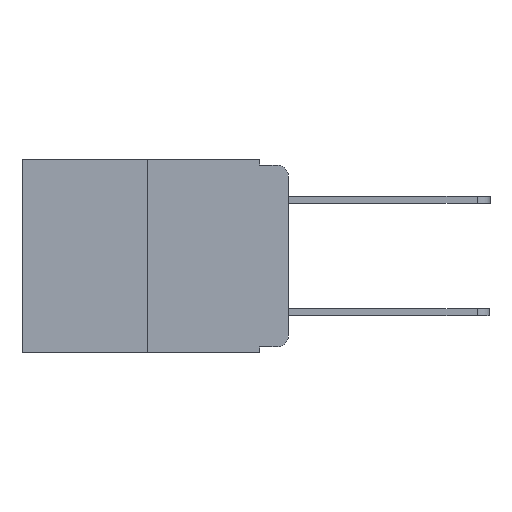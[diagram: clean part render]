
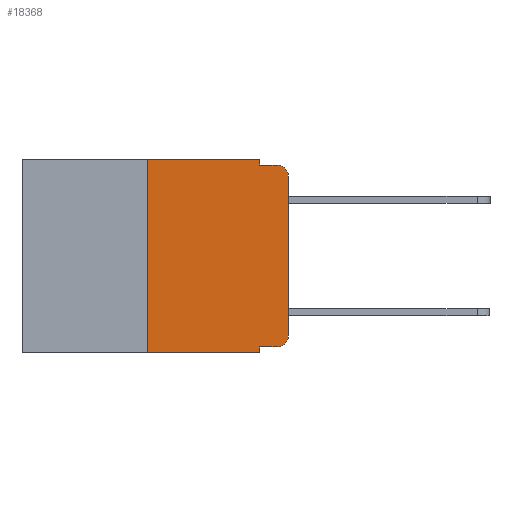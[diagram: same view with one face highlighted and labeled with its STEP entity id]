
A CAD part, left-side view. The second image highlights one B-rep face of the part: STEP entity #18368.
In plain terms, the highlighted planar face has unit normal (-1, 0, 0).
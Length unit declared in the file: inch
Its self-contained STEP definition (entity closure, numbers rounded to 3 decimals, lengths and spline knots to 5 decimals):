
#174 = LINE ( 'NONE', #11953, #8660 ) ;
#197 = DIRECTION ( 'NONE',  ( 0., -1., 0. ) ) ;
#627 = CIRCLE ( 'NONE', #7458, 0.02 ) ;
#633 = FACE_OUTER_BOUND ( 'NONE', #10012, .T. ) ;
#729 = EDGE_CURVE ( 'NONE', #17519, #19519, #13135, .T. ) ;
#1101 = AXIS2_PLACEMENT_3D ( 'NONE', #19298, #20832, #11351 ) ;
#1131 = VECTOR ( 'NONE', #9187, 39.37008 ) ;
#1470 = DIRECTION ( 'NONE',  ( 0., 0., 1. ) ) ;
#1717 = CARTESIAN_POINT ( 'NONE',  ( 0., 0.25, -0.343 ) ) ;
#2043 = ORIENTED_EDGE ( 'NONE', *, *, #7454, .F. ) ;
#2883 = LINE ( 'NONE', #11613, #15964 ) ;
#3343 = CARTESIAN_POINT ( 'NONE',  ( 0., 0.02, -0.03 ) ) ;
#3801 = EDGE_CURVE ( 'NONE', #7958, #6094, #5307, .T. ) ;
#4174 = EDGE_CURVE ( 'NONE', #19519, #8230, #627, .T. ) ;
#4401 = ORIENTED_EDGE ( 'NONE', *, *, #20935, .T. ) ;
#4832 = DIRECTION ( 'NONE',  ( 0., 0., 1. ) ) ;
#4846 = DIRECTION ( 'NONE',  ( -1., 0., 0. ) ) ;
#5013 = DIRECTION ( 'NONE',  ( 0., 0., -1. ) ) ;
#5307 = LINE ( 'NONE', #10705, #13522 ) ;
#5488 = VECTOR ( 'NONE', #1470, 39.37008 ) ;
#5568 = CARTESIAN_POINT ( 'NONE',  ( 0., 0., 0. ) ) ;
#5760 = DIRECTION ( 'NONE',  ( 0., -1., 0. ) ) ;
#5832 = CARTESIAN_POINT ( 'NONE',  ( 0., 0., -0.03 ) ) ;
#6094 = VERTEX_POINT ( 'NONE', #17076 ) ;
#6230 = EDGE_CURVE ( 'NONE', #17071, #16014, #14375, .T. ) ;
#7445 = ORIENTED_EDGE ( 'NONE', *, *, #14983, .F. ) ;
#7454 = EDGE_CURVE ( 'NONE', #19368, #8230, #174, .T. ) ;
#7458 = AXIS2_PLACEMENT_3D ( 'NONE', #3343, #14835, #5013 ) ;
#7958 = VERTEX_POINT ( 'NONE', #1717 ) ;
#8230 = VERTEX_POINT ( 'NONE', #19540 ) ;
#8660 = VECTOR ( 'NONE', #197, 39.37008 ) ;
#9187 = DIRECTION ( 'NONE',  ( 0., -1., 0. ) ) ;
#9272 = ORIENTED_EDGE ( 'NONE', *, *, #729, .T. ) ;
#9540 = ORIENTED_EDGE ( 'NONE', *, *, #14117, .F. ) ;
#9679 = PLANE ( 'NONE',  #1101 ) ;
#9696 = EDGE_CURVE ( 'NONE', #12415, #19368, #2883, .T. ) ;
#10012 = EDGE_LOOP ( 'NONE', ( #9272, #14179, #2043, #15160, #7445, #16662, #20772, #9540, #20092, #4401 ) ) ;
#10100 = DIRECTION ( 'NONE',  ( 0., -1., 0. ) ) ;
#10413 = DIRECTION ( 'NONE',  ( 0., 0., -1. ) ) ;
#10705 = CARTESIAN_POINT ( 'NONE',  ( 0., 0.473, -0.343 ) ) ;
#10852 = EDGE_CURVE ( 'NONE', #7958, #14284, #13707, .T. ) ;
#11351 = DIRECTION ( 'NONE',  ( 0., 0., -1. ) ) ;
#11410 = CARTESIAN_POINT ( 'NONE',  ( 0., 0.25, 0. ) ) ;
#11433 = CARTESIAN_POINT ( 'NONE',  ( 0., 0.25, 0. ) ) ;
#11593 = AXIS2_PLACEMENT_3D ( 'NONE', #14691, #4846, #16286 ) ;
#11613 = CARTESIAN_POINT ( 'NONE',  ( 0., 0.051, 0. ) ) ;
#11731 = CARTESIAN_POINT ( 'NONE',  ( 0., 0.473, 0. ) ) ;
#11953 = CARTESIAN_POINT ( 'NONE',  ( 0., 0.051, -0.01 ) ) ;
#12415 = VERTEX_POINT ( 'NONE', #20656 ) ;
#13135 = LINE ( 'NONE', #5568, #21039 ) ;
#13522 = VECTOR ( 'NONE', #5760, 39.37008 ) ;
#13707 = LINE ( 'NONE', #11433, #5488 ) ;
#14117 = EDGE_CURVE ( 'NONE', #17071, #6094, #15305, .T. ) ;
#14179 = ORIENTED_EDGE ( 'NONE', *, *, #4174, .T. ) ;
#14284 = VERTEX_POINT ( 'NONE', #11410 ) ;
#14375 = LINE ( 'NONE', #18825, #1131 ) ;
#14691 = CARTESIAN_POINT ( 'NONE',  ( 0., 0.02, -0.313 ) ) ;
#14778 = VECTOR ( 'NONE', #10100, 39.37008 ) ;
#14835 = DIRECTION ( 'NONE',  ( -1., 0., 0. ) ) ;
#14983 = EDGE_CURVE ( 'NONE', #14284, #12415, #18961, .T. ) ;
#15160 = ORIENTED_EDGE ( 'NONE', *, *, #9696, .F. ) ;
#15275 = CARTESIAN_POINT ( 'NONE',  ( 0., 0.051, -0.01 ) ) ;
#15305 = LINE ( 'NONE', #18366, #16307 ) ;
#15335 = CARTESIAN_POINT ( 'NONE',  ( 0., 0.051, -0.333 ) ) ;
#15964 = VECTOR ( 'NONE', #21103, 39.37008 ) ;
#16014 = VERTEX_POINT ( 'NONE', #18947 ) ;
#16286 = DIRECTION ( 'NONE',  ( 0., 0., -1. ) ) ;
#16307 = VECTOR ( 'NONE', #10413, 39.37008 ) ;
#16662 = ORIENTED_EDGE ( 'NONE', *, *, #10852, .F. ) ;
#16804 = CIRCLE ( 'NONE', #11593, 0.02 ) ;
#17071 = VERTEX_POINT ( 'NONE', #15335 ) ;
#17076 = CARTESIAN_POINT ( 'NONE',  ( 0., 0.051, -0.343 ) ) ;
#17519 = VERTEX_POINT ( 'NONE', #18639 ) ;
#18366 = CARTESIAN_POINT ( 'NONE',  ( 0., 0.051, 0. ) ) ;
#18368 = ADVANCED_FACE ( 'NONE', ( #633 ), #9679, .F. ) ;
#18639 = CARTESIAN_POINT ( 'NONE',  ( 0., 0., -0.313 ) ) ;
#18825 = CARTESIAN_POINT ( 'NONE',  ( 0., 0.051, -0.333 ) ) ;
#18947 = CARTESIAN_POINT ( 'NONE',  ( 0., 0.02, -0.333 ) ) ;
#18961 = LINE ( 'NONE', #11731, #14778 ) ;
#19298 = CARTESIAN_POINT ( 'NONE',  ( 0., 0.473, 0. ) ) ;
#19368 = VERTEX_POINT ( 'NONE', #15275 ) ;
#19519 = VERTEX_POINT ( 'NONE', #5832 ) ;
#19540 = CARTESIAN_POINT ( 'NONE',  ( 0., 0.02, -0.01 ) ) ;
#20092 = ORIENTED_EDGE ( 'NONE', *, *, #6230, .T. ) ;
#20656 = CARTESIAN_POINT ( 'NONE',  ( 0., 0.051, 0. ) ) ;
#20772 = ORIENTED_EDGE ( 'NONE', *, *, #3801, .T. ) ;
#20832 = DIRECTION ( 'NONE',  ( 1., 0., 0. ) ) ;
#20935 = EDGE_CURVE ( 'NONE', #16014, #17519, #16804, .T. ) ;
#21039 = VECTOR ( 'NONE', #4832, 39.37008 ) ;
#21103 = DIRECTION ( 'NONE',  ( 0., 0., -1. ) ) ;
